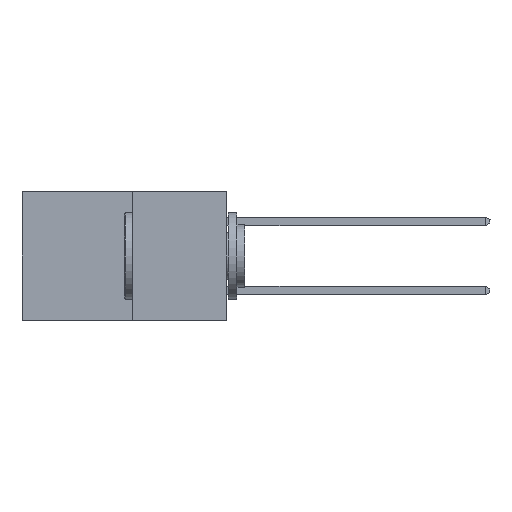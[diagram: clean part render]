
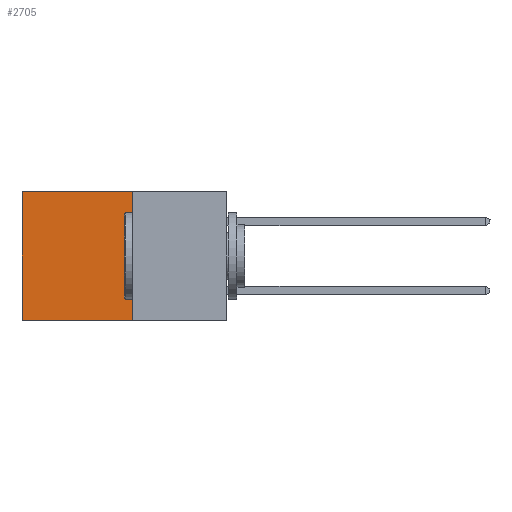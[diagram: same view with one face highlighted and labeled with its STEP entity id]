
A CAD part, left-side view. The second image highlights one B-rep face of the part: STEP entity #2705.
In plain terms, the highlighted planar face has unit normal (-1, 0, 0).
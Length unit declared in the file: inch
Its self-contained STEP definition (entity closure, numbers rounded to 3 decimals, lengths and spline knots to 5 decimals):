
#213 = VERTEX_POINT ( 'NONE', #9425 ) ;
#304 = AXIS2_PLACEMENT_3D ( 'NONE', #9311, #8922, #8893 ) ;
#1242 = CARTESIAN_POINT ( 'NONE',  ( 0.277, 0.27, 0. ) ) ;
#1527 = ORIENTED_EDGE ( 'NONE', *, *, #8132, .F. ) ;
#1559 = EDGE_CURVE ( 'NONE', #6153, #8636, #3996, .T. ) ;
#1706 = VECTOR ( 'NONE', #3073, 39.37008 ) ;
#2112 = ORIENTED_EDGE ( 'NONE', *, *, #1559, .T. ) ;
#2705 = ADVANCED_FACE ( 'NONE', ( #3759 ), #8940, .F. ) ;
#2781 = DIRECTION ( 'NONE',  ( 0., 0., -1. ) ) ;
#3073 = DIRECTION ( 'NONE',  ( 0., 1., 0. ) ) ;
#3304 = VECTOR ( 'NONE', #2781, 39.37008 ) ;
#3759 = FACE_OUTER_BOUND ( 'NONE', #9654, .T. ) ;
#3771 = EDGE_CURVE ( 'NONE', #213, #4699, #9035, .T. ) ;
#3996 = LINE ( 'NONE', #1242, #1706 ) ;
#4049 = VECTOR ( 'NONE', #6154, 39.37008 ) ;
#4619 = VECTOR ( 'NONE', #10683, 39.37008 ) ;
#4699 = VERTEX_POINT ( 'NONE', #9102 ) ;
#4939 = CARTESIAN_POINT ( 'NONE',  ( 0.277, 0.59, 0. ) ) ;
#5584 = CARTESIAN_POINT ( 'NONE',  ( 0.277, 0.27, 0. ) ) ;
#5710 = EDGE_CURVE ( 'NONE', #8636, #4699, #7917, .T. ) ;
#6003 = CARTESIAN_POINT ( 'NONE',  ( 0.277, 0.59, -0.37 ) ) ;
#6153 = VERTEX_POINT ( 'NONE', #5584 ) ;
#6154 = DIRECTION ( 'NONE',  ( 0., 0., -1. ) ) ;
#7664 = ORIENTED_EDGE ( 'NONE', *, *, #3771, .F. ) ;
#7917 = LINE ( 'NONE', #6003, #3304 ) ;
#8132 = EDGE_CURVE ( 'NONE', #6153, #213, #8413, .T. ) ;
#8209 = CARTESIAN_POINT ( 'NONE',  ( 0.277, 0.27, -0.37 ) ) ;
#8413 = LINE ( 'NONE', #10306, #4049 ) ;
#8636 = VERTEX_POINT ( 'NONE', #4939 ) ;
#8893 = DIRECTION ( 'NONE',  ( 0., 0., -1. ) ) ;
#8922 = DIRECTION ( 'NONE',  ( 1., 0., 0. ) ) ;
#8940 = PLANE ( 'NONE',  #304 ) ;
#9035 = LINE ( 'NONE', #8209, #4619 ) ;
#9102 = CARTESIAN_POINT ( 'NONE',  ( 0.277, 0.59, -0.37 ) ) ;
#9311 = CARTESIAN_POINT ( 'NONE',  ( 0.277, 0.27, -0.37 ) ) ;
#9425 = CARTESIAN_POINT ( 'NONE',  ( 0.277, 0.27, -0.37 ) ) ;
#9654 = EDGE_LOOP ( 'NONE', ( #10772, #7664, #1527, #2112 ) ) ;
#10306 = CARTESIAN_POINT ( 'NONE',  ( 0.277, 0.27, -0.37 ) ) ;
#10683 = DIRECTION ( 'NONE',  ( 0., 1., 0. ) ) ;
#10772 = ORIENTED_EDGE ( 'NONE', *, *, #5710, .T. ) ;
